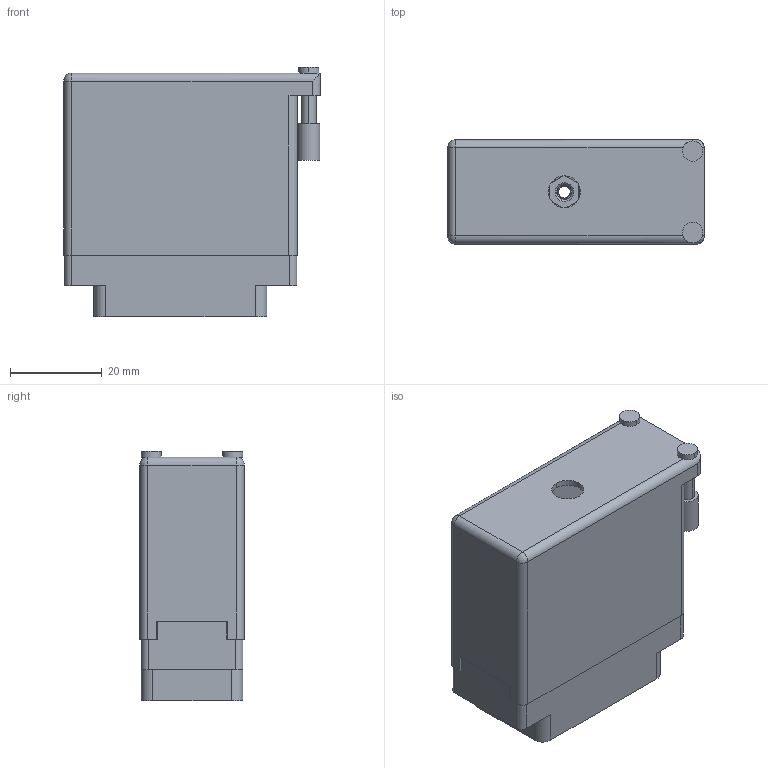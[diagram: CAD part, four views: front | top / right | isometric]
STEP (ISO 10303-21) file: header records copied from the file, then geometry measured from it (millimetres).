
FILE_DESCRIPTION (( 'STEP AP203' ), '1' );
FILE_NAME ('519-036-000-356.STEP', '2020-03-02T21:37:09', ( '' ), ( '' ), 'SwSTEP 2.0', 'SolidWorks 2016', '' );
FILE_SCHEMA (( 'CONFIG_CONTROL_DESIGN' ));
Length unit declared in the file: inch
Products named in the file (4): 516-252-035-100_516-252-035-100; 519-036-000-356; 519 Plug Insulator_036; 516-230-001_Metal - 038 Side Entry
Assembly tree (3 placements, depth 2):
  519-036-000-356
    519 Plug Insulator_036
    516-252-035-100_516-252-035-100
    516-230-001_Metal - 038 Side Entry
Bounding box: 56.08 x 22.83 x 54.51 mm (x, y, z)
Volume: 17840.8 mm3; surface area: 25268 mm2
Topology: 3 solids, 3 shells, 970 faces, 2812 edges, 1866 vertices
Faces by surface type: plane 659, cylinder 291, cone 12, bspline 6, sphere 2
Entity records: 34860 total; most frequent: CARTESIAN_POINT 8139, ORIENTED_EDGE 5620, DIRECTION 5406, EDGE_CURVE 2810, VECTOR 2044, LINE 2044, VERTEX_POINT 1866, AXIS2_PLACEMENT_3D 1681
